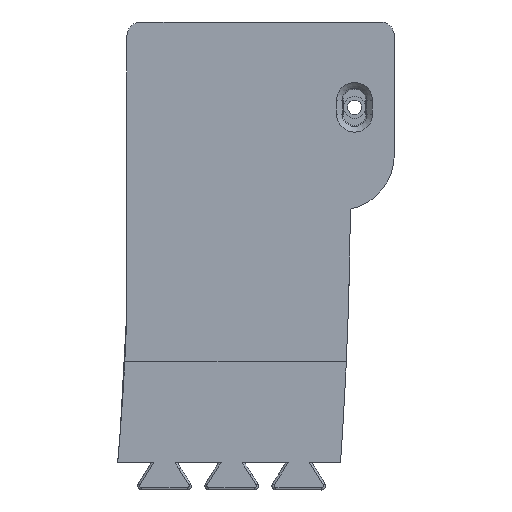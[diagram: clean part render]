
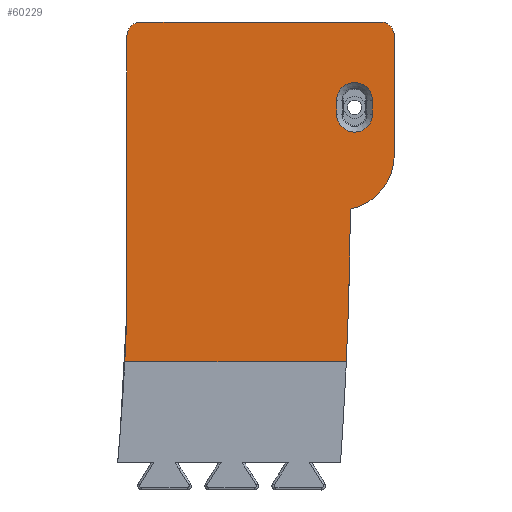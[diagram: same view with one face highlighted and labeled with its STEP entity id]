
A CAD part, front view. The second image highlights one B-rep face of the part: STEP entity #60229.
In plain terms, the highlighted planar face has unit normal (0, -1, 0).
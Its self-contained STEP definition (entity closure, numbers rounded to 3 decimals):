
#715=FACE_BOUND('',#13339,.T.);
#6491=CIRCLE('',#61588,949.);
#6506=CIRCLE('',#61615,1465.281);
#6507=CIRCLE('',#61631,5.);
#6508=CIRCLE('',#61632,20.);
#6509=CIRCLE('',#61633,5.);
#6510=CIRCLE('',#61634,6.439);
#6511=CIRCLE('',#61635,6.439);
#9771=FACE_OUTER_BOUND('',#13338,.T.);
#13338=EDGE_LOOP('',(#55574,#55575,#55576,#55577,#55578,#55579,#55580,#55581,
#55582,#55583));
#13339=EDGE_LOOP('',(#55584,#55585,#55586,#55587));
#14233=LINE('',#69114,#18394);
#14800=LINE('',#72002,#18961);
#18175=LINE('',#118689,#22336);
#18176=LINE('',#118692,#22337);
#18177=LINE('',#118696,#22338);
#18178=LINE('',#118699,#22339);
#18179=LINE('',#118703,#22340);
#18394=VECTOR('',#61890,10.);
#18961=VECTOR('',#62809,10.);
#22336=VECTOR('',#68330,10.);
#22337=VECTOR('',#68333,10.);
#22338=VECTOR('',#68338,10.);
#22339=VECTOR('',#68339,10.);
#22340=VECTOR('',#68342,10.);
#22944=VERTEX_POINT('',#69112);
#22945=VERTEX_POINT('',#69113);
#23466=VERTEX_POINT('',#71998);
#23468=VERTEX_POINT('',#72001);
#28720=VERTEX_POINT('',#118297);
#28749=VERTEX_POINT('',#118657);
#28750=VERTEX_POINT('',#118687);
#28751=VERTEX_POINT('',#118688);
#28752=VERTEX_POINT('',#118690);
#28753=VERTEX_POINT('',#118694);
#28754=VERTEX_POINT('',#118697);
#28755=VERTEX_POINT('',#118698);
#28756=VERTEX_POINT('',#118700);
#28757=VERTEX_POINT('',#118702);
#28978=EDGE_CURVE('',#22944,#22945,#14233,.T.);
#29757=EDGE_CURVE('',#23466,#23468,#14800,.T.);
#37668=EDGE_CURVE('',#28720,#22944,#6491,.T.);
#37714=EDGE_CURVE('',#22945,#28749,#6506,.T.);
#37727=EDGE_CURVE('',#28750,#28751,#18175,.T.);
#37728=EDGE_CURVE('',#28752,#28750,#6507,.T.);
#37729=EDGE_CURVE('',#28752,#28720,#18176,.T.);
#37730=EDGE_CURVE('',#23468,#28749,#6508,.T.);
#37731=EDGE_CURVE('',#28753,#23466,#6509,.T.);
#37732=EDGE_CURVE('',#28751,#28753,#18177,.T.);
#37733=EDGE_CURVE('',#28754,#28755,#18178,.T.);
#37734=EDGE_CURVE('',#28755,#28756,#6510,.T.);
#37735=EDGE_CURVE('',#28756,#28757,#18179,.T.);
#37736=EDGE_CURVE('',#28757,#28754,#6511,.T.);
#55574=ORIENTED_EDGE('',*,*,#37727,.F.);
#55575=ORIENTED_EDGE('',*,*,#37728,.F.);
#55576=ORIENTED_EDGE('',*,*,#37729,.T.);
#55577=ORIENTED_EDGE('',*,*,#37668,.T.);
#55578=ORIENTED_EDGE('',*,*,#28978,.T.);
#55579=ORIENTED_EDGE('',*,*,#37714,.T.);
#55580=ORIENTED_EDGE('',*,*,#37730,.F.);
#55581=ORIENTED_EDGE('',*,*,#29757,.F.);
#55582=ORIENTED_EDGE('',*,*,#37731,.F.);
#55583=ORIENTED_EDGE('',*,*,#37732,.F.);
#55584=ORIENTED_EDGE('',*,*,#37733,.T.);
#55585=ORIENTED_EDGE('',*,*,#37734,.T.);
#55586=ORIENTED_EDGE('',*,*,#37735,.T.);
#55587=ORIENTED_EDGE('',*,*,#37736,.T.);
#56975=PLANE('',#61630);
#60229=ADVANCED_FACE('',(#9771,#715),#56975,.T.);
#61588=AXIS2_PLACEMENT_3D('',#118298,#68220,#68221);
#61615=AXIS2_PLACEMENT_3D('',#118659,#68286,#68287);
#61630=AXIS2_PLACEMENT_3D('',#118686,#68328,#68329);
#61631=AXIS2_PLACEMENT_3D('',#118691,#68331,#68332);
#61632=AXIS2_PLACEMENT_3D('',#118693,#68334,#68335);
#61633=AXIS2_PLACEMENT_3D('',#118695,#68336,#68337);
#61634=AXIS2_PLACEMENT_3D('',#118701,#68340,#68341);
#61635=AXIS2_PLACEMENT_3D('',#118704,#68343,#68344);
#61890=DIRECTION('',(1.,0.,0.));
#62809=DIRECTION('',(0.,0.,-1.));
#68220=DIRECTION('center_axis',(0.,1.,0.));
#68221=DIRECTION('ref_axis',(1.,0.,-0.031));
#68286=DIRECTION('center_axis',(0.,-1.,0.));
#68287=DIRECTION('ref_axis',(1.,0.,-0.008));
#68328=DIRECTION('center_axis',(0.,-1.,0.));
#68329=DIRECTION('ref_axis',(1.,0.,0.));
#68330=DIRECTION('',(1.,0.,0.));
#68331=DIRECTION('center_axis',(0.,1.,0.));
#68332=DIRECTION('ref_axis',(-0.707,0.,0.707));
#68333=DIRECTION('',(0.,0.,-1.));
#68334=DIRECTION('center_axis',(0.,1.,0.));
#68335=DIRECTION('ref_axis',(0.208,0.,-0.978));
#68336=DIRECTION('center_axis',(0.,1.,0.));
#68337=DIRECTION('ref_axis',(0.707,0.,0.707));
#68338=DIRECTION('',(1.,0.,0.));
#68339=DIRECTION('',(0.,0.,1.));
#68340=DIRECTION('center_axis',(0.,1.,0.));
#68341=DIRECTION('ref_axis',(1.,0.,0.));
#68342=DIRECTION('',(0.,0.,-1.));
#68343=DIRECTION('center_axis',(0.,1.,0.));
#68344=DIRECTION('ref_axis',(-1.,0.,0.));
#69112=CARTESIAN_POINT('',(-101.234,6.118,-44.965));
#69113=CARTESIAN_POINT('',(-21.454,6.118,-44.965));
#69114=CARTESIAN_POINT('',(-106.432,6.118,-44.965));
#71998=CARTESIAN_POINT('',(-4.16,6.118,72.408));
#72001=CARTESIAN_POINT('',(-4.16,6.118,29.563));
#72002=CARTESIAN_POINT('',(-4.16,6.118,-37.278));
#118297=CARTESIAN_POINT('',(-100.44,6.118,-25.509));
#118298=CARTESIAN_POINT('Origin',(-1048.998,6.118,3.472));
#118657=CARTESIAN_POINT('',(-20.,6.118,10.));
#118659=CARTESIAN_POINT('Origin',(-1485.238,6.118,21.265));
#118686=CARTESIAN_POINT('Origin',(-73.595,6.118,-92.256));
#118687=CARTESIAN_POINT('',(-95.44,6.118,77.408));
#118688=CARTESIAN_POINT('',(-91.44,6.118,77.408));
#118689=CARTESIAN_POINT('',(-91.44,6.118,77.408));
#118690=CARTESIAN_POINT('',(-100.44,6.118,72.408));
#118691=CARTESIAN_POINT('Origin',(-95.44,6.118,72.408));
#118692=CARTESIAN_POINT('',(-100.44,6.118,14.491));
#118693=CARTESIAN_POINT('Origin',(-24.16,6.118,29.563));
#118694=CARTESIAN_POINT('',(-9.16,6.118,77.408));
#118695=CARTESIAN_POINT('Origin',(-9.16,6.118,72.408));
#118696=CARTESIAN_POINT('',(-9.16,6.118,77.408));
#118697=CARTESIAN_POINT('',(-24.93,6.118,44.172));
#118698=CARTESIAN_POINT('',(-24.93,6.118,49.176));
#118699=CARTESIAN_POINT('',(-24.93,6.118,65.879));
#118700=CARTESIAN_POINT('',(-12.053,6.118,49.176));
#118701=CARTESIAN_POINT('Origin',(-18.491,6.118,49.176));
#118702=CARTESIAN_POINT('',(-12.053,6.118,44.172));
#118703=CARTESIAN_POINT('',(-12.053,6.118,68.38));
#118704=CARTESIAN_POINT('Origin',(-18.491,6.118,44.172));
